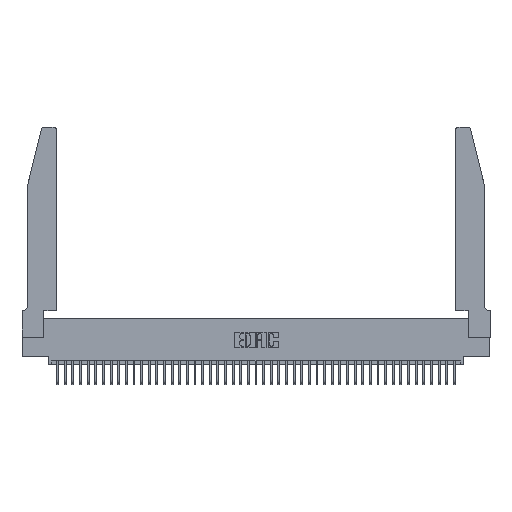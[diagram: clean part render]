
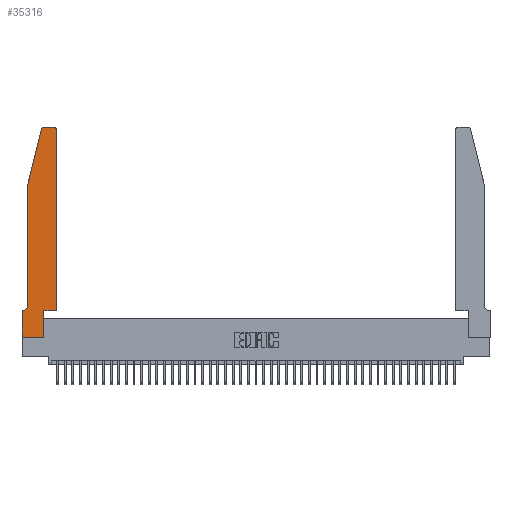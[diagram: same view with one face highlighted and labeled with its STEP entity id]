
A CAD part, top view. The second image highlights one B-rep face of the part: STEP entity #35316.
In plain terms, the highlighted planar face has unit normal (0, 0, 1).
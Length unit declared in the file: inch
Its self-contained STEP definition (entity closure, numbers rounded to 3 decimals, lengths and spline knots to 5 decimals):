
#621 = EDGE_CURVE ( 'NONE', #38567, #1329, #18119, .T. ) ;
#1130 = CARTESIAN_POINT ( 'NONE',  ( 0.4505, 0.35, 0.37 ) ) ;
#1329 = VERTEX_POINT ( 'NONE', #32954 ) ;
#1983 = VECTOR ( 'NONE', #21904, 39.37008 ) ;
#2370 = LINE ( 'NONE', #29125, #28054 ) ;
#2589 = VERTEX_POINT ( 'NONE', #17050 ) ;
#2751 = VECTOR ( 'NONE', #11059, 39.37008 ) ;
#3262 = EDGE_CURVE ( 'NONE', #14861, #22450, #40399, .T. ) ;
#3331 = EDGE_CURVE ( 'NONE', #2589, #38567, #28415, .T. ) ;
#3796 = AXIS2_PLACEMENT_3D ( 'NONE', #27989, #8109, #31319 ) ;
#4423 = CARTESIAN_POINT ( 'NONE',  ( 0.2605, 2.75, 0.37 ) ) ;
#5022 = EDGE_CURVE ( 'NONE', #11779, #30134, #36569, .T. ) ;
#5131 = CARTESIAN_POINT ( 'NONE',  ( 0., 0., 0.37 ) ) ;
#5321 = CARTESIAN_POINT ( 'NONE',  ( 0.284, 2.72, 0.37 ) ) ;
#6870 = ORIENTED_EDGE ( 'NONE', *, *, #32414, .T. ) ;
#7707 = CARTESIAN_POINT ( 'NONE',  ( 0., 0.35, 0.37 ) ) ;
#8109 = DIRECTION ( 'NONE',  ( 0., 0., 1. ) ) ;
#8223 = EDGE_CURVE ( 'NONE', #30134, #24262, #2370, .T. ) ;
#8512 = LINE ( 'NONE', #33761, #25095 ) ;
#8739 = CARTESIAN_POINT ( 'NONE',  ( 0.0755, 2., 0.37 ) ) ;
#8753 = DIRECTION ( 'NONE',  ( 1., 0., 0. ) ) ;
#10356 = VECTOR ( 'NONE', #12960, 39.37008 ) ;
#11059 = DIRECTION ( 'NONE',  ( 1., 0., 0. ) ) ;
#11732 = EDGE_CURVE ( 'NONE', #31134, #11779, #12277, .T. ) ;
#11779 = VERTEX_POINT ( 'NONE', #37951 ) ;
#12277 = LINE ( 'NONE', #4423, #29931 ) ;
#12344 = CARTESIAN_POINT ( 'NONE',  ( 0.25487, 2.72718, 0.37 ) ) ;
#12960 = DIRECTION ( 'NONE',  ( 0., 1., 0. ) ) ;
#13378 = EDGE_CURVE ( 'NONE', #21521, #41099, #8512, .T. ) ;
#13454 = DIRECTION ( 'NONE',  ( 0., -1., 0. ) ) ;
#13582 = AXIS2_PLACEMENT_3D ( 'NONE', #18849, #42116, #22154 ) ;
#13879 = VECTOR ( 'NONE', #27149, 39.37008 ) ;
#14861 = VERTEX_POINT ( 'NONE', #5131 ) ;
#15253 = CARTESIAN_POINT ( 'NONE',  ( 0.0055, 0.35, 0.37 ) ) ;
#15601 = ORIENTED_EDGE ( 'NONE', *, *, #30070, .T. ) ;
#16344 = CARTESIAN_POINT ( 'NONE',  ( 0., 0.35, 0.37 ) ) ;
#17050 = CARTESIAN_POINT ( 'NONE',  ( 0.2865, 0.35, 0.37 ) ) ;
#17107 = ORIENTED_EDGE ( 'NONE', *, *, #24871, .T. ) ;
#18119 = LINE ( 'NONE', #29153, #10356 ) ;
#18849 = CARTESIAN_POINT ( 'NONE',  ( 0.0055, 0.42, 0.37 ) ) ;
#18885 = AXIS2_PLACEMENT_3D ( 'NONE', #5321, #28619, #8753 ) ;
#19104 = LINE ( 'NONE', #25228, #26928 ) ;
#19661 = DIRECTION ( 'NONE',  ( 1., 0., 0. ) ) ;
#19738 = ORIENTED_EDGE ( 'NONE', *, *, #8223, .T. ) ;
#19851 = LINE ( 'NONE', #8739, #1983 ) ;
#21521 = VERTEX_POINT ( 'NONE', #15253 ) ;
#21904 = DIRECTION ( 'NONE',  ( 0., -1., 0. ) ) ;
#22154 = DIRECTION ( 'NONE',  ( -1., 0., 0. ) ) ;
#22296 = EDGE_CURVE ( 'NONE', #41099, #14861, #36945, .T. ) ;
#22362 = VECTOR ( 'NONE', #13454, 39.37008 ) ;
#22450 = VERTEX_POINT ( 'NONE', #27228 ) ;
#23774 = CARTESIAN_POINT ( 'NONE',  ( 0., 0., 0.37 ) ) ;
#24262 = VERTEX_POINT ( 'NONE', #28783 ) ;
#24423 = DIRECTION ( 'NONE',  ( -1., 0., 0. ) ) ;
#24871 = EDGE_CURVE ( 'NONE', #22450, #2589, #19104, .T. ) ;
#25095 = VECTOR ( 'NONE', #37102, 39.37008 ) ;
#25162 = CARTESIAN_POINT ( 'NONE',  ( 0.0755, 0.42, 0.37 ) ) ;
#25228 = CARTESIAN_POINT ( 'NONE',  ( 0.2865, 0.35, 0.37 ) ) ;
#25485 = ORIENTED_EDGE ( 'NONE', *, *, #3262, .T. ) ;
#26587 = EDGE_CURVE ( 'NONE', #35706, #21521, #37682, .T. ) ;
#26928 = VECTOR ( 'NONE', #35107, 39.37008 ) ;
#27149 = DIRECTION ( 'NONE',  ( 1., 0., 0. ) ) ;
#27228 = CARTESIAN_POINT ( 'NONE',  ( 0.2865, 0., 0.37 ) ) ;
#27989 = CARTESIAN_POINT ( 'NONE',  ( 0.4205, 2.72, 0.37 ) ) ;
#28054 = VECTOR ( 'NONE', #39024, 39.37008 ) ;
#28415 = LINE ( 'NONE', #30908, #2751 ) ;
#28619 = DIRECTION ( 'NONE',  ( 0., 0., 1. ) ) ;
#28783 = CARTESIAN_POINT ( 'NONE',  ( 0.0755, 2., 0.37 ) ) ;
#29125 = CARTESIAN_POINT ( 'NONE',  ( 0.0755, 2., 0.37 ) ) ;
#29153 = CARTESIAN_POINT ( 'NONE',  ( 0.4505, 0.35, 0.37 ) ) ;
#29293 = ORIENTED_EDGE ( 'NONE', *, *, #22296, .T. ) ;
#29559 = PLANE ( 'NONE',  #42470 ) ;
#29931 = VECTOR ( 'NONE', #24423, 39.37008 ) ;
#30070 = EDGE_CURVE ( 'NONE', #24262, #35706, #19851, .T. ) ;
#30134 = VERTEX_POINT ( 'NONE', #12344 ) ;
#30908 = CARTESIAN_POINT ( 'NONE',  ( 0.4505, 0.35, 0.37 ) ) ;
#30950 = ORIENTED_EDGE ( 'NONE', *, *, #621, .T. ) ;
#31134 = VERTEX_POINT ( 'NONE', #34190 ) ;
#31319 = DIRECTION ( 'NONE',  ( 1., 0., 0. ) ) ;
#31758 = ORIENTED_EDGE ( 'NONE', *, *, #3331, .T. ) ;
#32095 = CIRCLE ( 'NONE', #3796, 0.03 ) ;
#32285 = ORIENTED_EDGE ( 'NONE', *, *, #13378, .T. ) ;
#32414 = EDGE_CURVE ( 'NONE', #1329, #31134, #32095, .T. ) ;
#32954 = CARTESIAN_POINT ( 'NONE',  ( 0.4505, 2.72, 0.37 ) ) ;
#33312 = CARTESIAN_POINT ( 'NONE',  ( 0., 0., 0.37 ) ) ;
#33761 = CARTESIAN_POINT ( 'NONE',  ( 0.0755, 0.35, 0.37 ) ) ;
#34190 = CARTESIAN_POINT ( 'NONE',  ( 0.4205, 2.75, 0.37 ) ) ;
#35107 = DIRECTION ( 'NONE',  ( 0., 1., 0. ) ) ;
#35316 = ADVANCED_FACE ( 'NONE', ( #37147 ), #29559, .T. ) ;
#35706 = VERTEX_POINT ( 'NONE', #25162 ) ;
#36569 = CIRCLE ( 'NONE', #18885, 0.03 ) ;
#36945 = LINE ( 'NONE', #33312, #22362 ) ;
#36984 = ORIENTED_EDGE ( 'NONE', *, *, #5022, .T. ) ;
#37102 = DIRECTION ( 'NONE',  ( -1., 0., 0. ) ) ;
#37147 = FACE_OUTER_BOUND ( 'NONE', #43147, .T. ) ;
#37307 = ORIENTED_EDGE ( 'NONE', *, *, #26587, .T. ) ;
#37682 = CIRCLE ( 'NONE', #13582, 0.07 ) ;
#37951 = CARTESIAN_POINT ( 'NONE',  ( 0.284, 2.75, 0.37 ) ) ;
#38567 = VERTEX_POINT ( 'NONE', #1130 ) ;
#39024 = DIRECTION ( 'NONE',  ( -0.239, -0.971, 0. ) ) ;
#39614 = DIRECTION ( 'NONE',  ( 0., 0., 1. ) ) ;
#40189 = ORIENTED_EDGE ( 'NONE', *, *, #11732, .T. ) ;
#40399 = LINE ( 'NONE', #23774, #13879 ) ;
#41099 = VERTEX_POINT ( 'NONE', #7707 ) ;
#42116 = DIRECTION ( 'NONE',  ( 0., 0., -1. ) ) ;
#42470 = AXIS2_PLACEMENT_3D ( 'NONE', #16344, #39614, #19661 ) ;
#43147 = EDGE_LOOP ( 'NONE', ( #40189, #36984, #19738, #15601, #37307, #32285, #29293, #25485, #17107, #31758, #30950, #6870 ) ) ;
